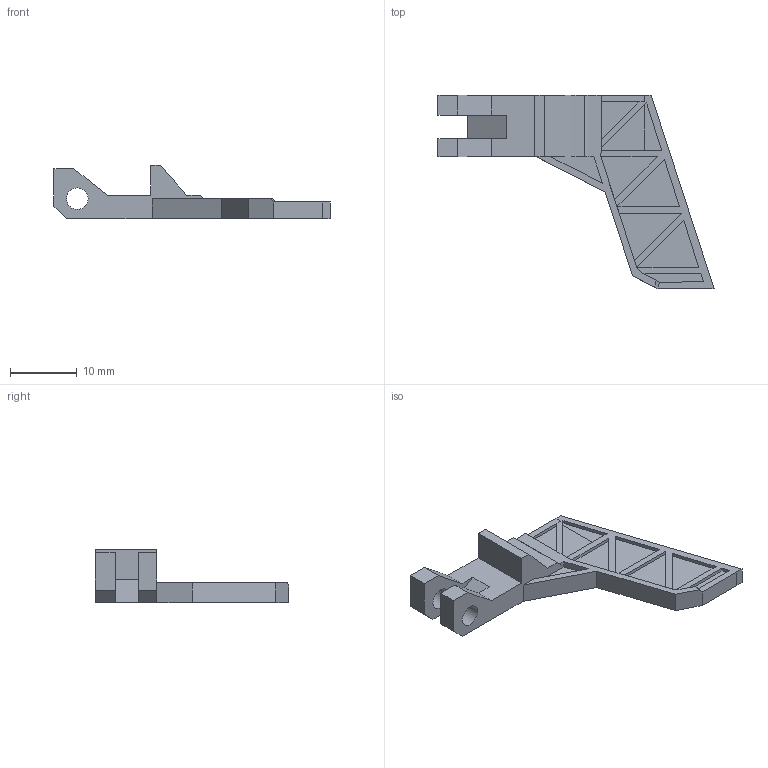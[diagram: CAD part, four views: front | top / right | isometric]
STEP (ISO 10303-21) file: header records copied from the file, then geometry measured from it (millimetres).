
FILE_DESCRIPTION(/* description */ (''),/* implementation_level */ '2;1');
FILE_NAME(/* name */ 'latte wing.step',/* time_stamp */ '2021-05-31T19:22:38-06:00',/* author */ (''),/* organization */ (''),/* preprocessor_version */ 'ST-DEVELOPER v18.1',/* originating_system */ 'Autodesk Translation Framework v10.9.0.1377',/* authorisation */ '');
FILE_SCHEMA (('AUTOMOTIVE_DESIGN { 1 0 10303 214 3 1 1 }'));
Length unit declared in the file: millimetre
Products named in the file (1): MAC bar mag release
Bounding box: 41.46 x 29.04 x 8 mm (x, y, z)
Volume: 1655.2 mm3; surface area: 1851.9 mm2
Topology: 1 solids, 1 shells, 71 faces, 194 edges, 125 vertices
Faces by surface type: plane 69, cylinder 2
Full cylindrical faces by diameter (mm): 3.25 x2
Entity records: 2229 total; most frequent: CARTESIAN_POINT 391, ORIENTED_EDGE 388, DIRECTION 342, EDGE_CURVE 194, LINE 190, VECTOR 190, VERTEX_POINT 125, AXIS2_PLACEMENT_3D 76
